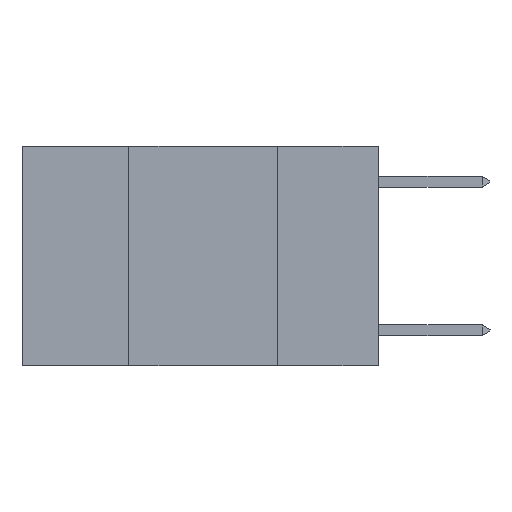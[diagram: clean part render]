
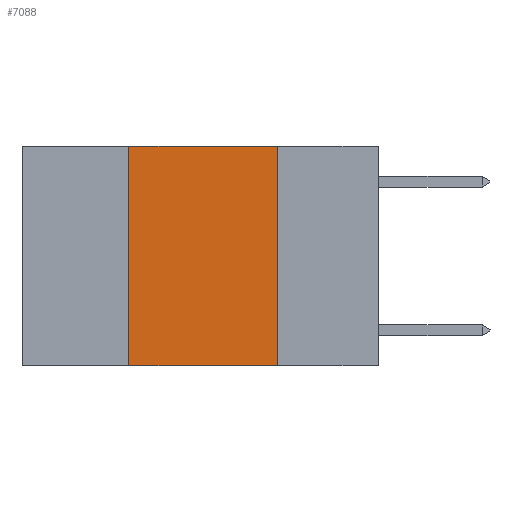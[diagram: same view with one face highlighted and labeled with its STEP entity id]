
A CAD part, left-side view. The second image highlights one B-rep face of the part: STEP entity #7088.
In plain terms, the highlighted planar face has unit normal (-1, 0, 0).
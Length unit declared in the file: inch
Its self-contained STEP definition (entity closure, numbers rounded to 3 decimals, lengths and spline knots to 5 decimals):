
#28 = DIRECTION ( 'NONE',  ( 0., -1., 0. ) ) ;
#1288 = EDGE_CURVE ( 'NONE', #13595, #22484, #9939, .T. ) ;
#1758 = CARTESIAN_POINT ( 'NONE',  ( 0., 0.42, 0. ) ) ;
#2580 = VECTOR ( 'NONE', #28, 39.37008 ) ;
#2805 = ORIENTED_EDGE ( 'NONE', *, *, #16077, .F. ) ;
#3163 = ORIENTED_EDGE ( 'NONE', *, *, #13900, .F. ) ;
#3400 = ORIENTED_EDGE ( 'NONE', *, *, #15525, .F. ) ;
#3457 = ORIENTED_EDGE ( 'NONE', *, *, #1288, .T. ) ;
#3916 = DIRECTION ( 'NONE',  ( 0., 0., -1. ) ) ;
#3987 = EDGE_LOOP ( 'NONE', ( #2805, #3163, #3400, #3457 ) ) ;
#5419 = VERTEX_POINT ( 'NONE', #1758 ) ;
#5429 = DIRECTION ( 'NONE',  ( 0., 0., -1. ) ) ;
#5846 = CARTESIAN_POINT ( 'NONE',  ( 0., 0.17, 0. ) ) ;
#7088 = ADVANCED_FACE ( 'NONE', ( #11169 ), #12785, .F. ) ;
#9939 = LINE ( 'NONE', #10322, #23944 ) ;
#10322 = CARTESIAN_POINT ( 'NONE',  ( 0., 0.6, -0.37 ) ) ;
#11169 = FACE_OUTER_BOUND ( 'NONE', #3987, .T. ) ;
#11377 = CARTESIAN_POINT ( 'NONE',  ( 0., 0.6, 0. ) ) ;
#11398 = VECTOR ( 'NONE', #3916, 39.37008 ) ;
#12785 = PLANE ( 'NONE',  #17769 ) ;
#13279 = CARTESIAN_POINT ( 'NONE',  ( 0., 0.17, -0.37 ) ) ;
#13595 = VERTEX_POINT ( 'NONE', #23313 ) ;
#13900 = EDGE_CURVE ( 'NONE', #5419, #16504, #16913, .T. ) ;
#14335 = CARTESIAN_POINT ( 'NONE',  ( 0., 0.17, 0. ) ) ;
#14649 = CARTESIAN_POINT ( 'NONE',  ( 0., 0.6, 0. ) ) ;
#15525 = EDGE_CURVE ( 'NONE', #13595, #5419, #19249, .T. ) ;
#15573 = DIRECTION ( 'NONE',  ( 0., -1., 0. ) ) ;
#16077 = EDGE_CURVE ( 'NONE', #16504, #22484, #16911, .T. ) ;
#16504 = VERTEX_POINT ( 'NONE', #14335 ) ;
#16545 = DIRECTION ( 'NONE',  ( 1., 0., 0. ) ) ;
#16911 = LINE ( 'NONE', #5846, #11398 ) ;
#16913 = LINE ( 'NONE', #11377, #2580 ) ;
#17769 = AXIS2_PLACEMENT_3D ( 'NONE', #14649, #16545, #5429 ) ;
#19249 = LINE ( 'NONE', #20934, #23995 ) ;
#20934 = CARTESIAN_POINT ( 'NONE',  ( 0., 0.42, 0. ) ) ;
#22484 = VERTEX_POINT ( 'NONE', #13279 ) ;
#22748 = DIRECTION ( 'NONE',  ( 0., 0., 1. ) ) ;
#23313 = CARTESIAN_POINT ( 'NONE',  ( 0., 0.42, -0.37 ) ) ;
#23944 = VECTOR ( 'NONE', #15573, 39.37008 ) ;
#23995 = VECTOR ( 'NONE', #22748, 39.37008 ) ;
